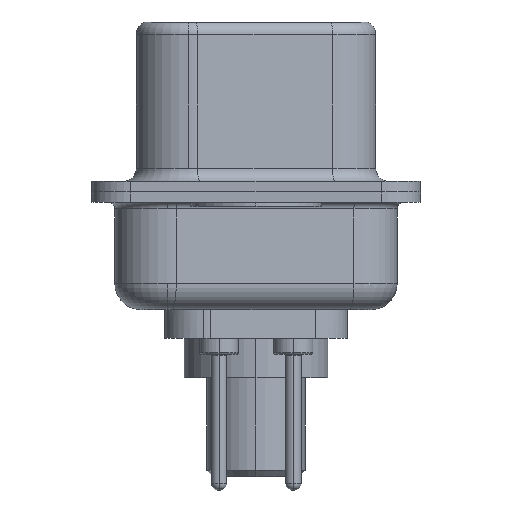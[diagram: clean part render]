
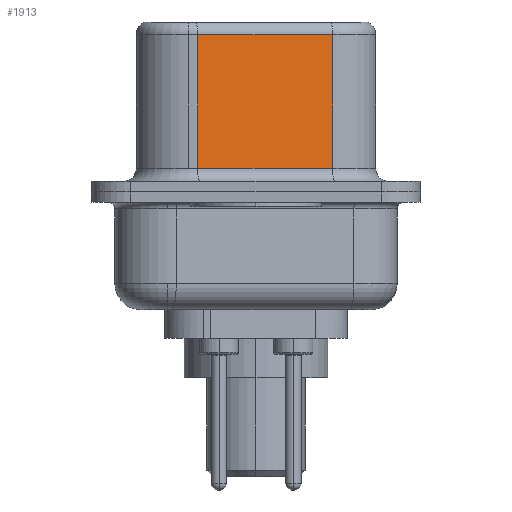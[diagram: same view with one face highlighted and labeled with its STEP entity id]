
A CAD part, left-side view. The second image highlights one B-rep face of the part: STEP entity #1913.
In plain terms, the highlighted planar face has unit normal (-0.985, -0.174, 0).
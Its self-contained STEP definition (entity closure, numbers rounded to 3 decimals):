
#334 = CARTESIAN_POINT ( 'NONE',  ( 3.67, 2.233, 6.02 ) ) ;
#497 = VECTOR ( 'NONE', #7940, 1000. ) ;
#1575 = AXIS2_PLACEMENT_3D ( 'NONE', #11495, #7559, #7485 ) ;
#1751 = VECTOR ( 'NONE', #2041, 1000. ) ;
#1789 = EDGE_CURVE ( 'NONE', #7858, #7710, #10670, .T. ) ;
#1827 = CARTESIAN_POINT ( 'NONE',  ( 4.58, -2.927, 0.9 ) ) ;
#1913 = ADVANCED_FACE ( 'NONE', ( #11664 ), #5556, .F. ) ;
#1963 = EDGE_CURVE ( 'NONE', #10136, #7858, #3935, .T. ) ;
#2041 = DIRECTION ( 'NONE',  ( 0., 0., -1. ) ) ;
#2373 = ORIENTED_EDGE ( 'NONE', *, *, #1963, .T. ) ;
#3032 = LINE ( 'NONE', #3913, #497 ) ;
#3173 = ORIENTED_EDGE ( 'NONE', *, *, #1789, .T. ) ;
#3664 = ORIENTED_EDGE ( 'NONE', *, *, #6048, .F. ) ;
#3708 = DIRECTION ( 'NONE',  ( -0.174, 0.985, 0. ) ) ;
#3713 = ORIENTED_EDGE ( 'NONE', *, *, #5382, .T. ) ;
#3913 = CARTESIAN_POINT ( 'NONE',  ( 4.58, -2.927, 6.52 ) ) ;
#3935 = LINE ( 'NONE', #6809, #1751 ) ;
#5369 = DIRECTION ( 'NONE',  ( 0.174, -0.985, 0. ) ) ;
#5382 = EDGE_CURVE ( 'NONE', #8556, #10136, #6538, .T. ) ;
#5556 = PLANE ( 'NONE',  #1575 ) ;
#6048 = EDGE_CURVE ( 'NONE', #8556, #7710, #3032, .T. ) ;
#6114 = CARTESIAN_POINT ( 'NONE',  ( 3.67, 2.233, 0.9 ) ) ;
#6538 = LINE ( 'NONE', #8829, #8767 ) ;
#6809 = CARTESIAN_POINT ( 'NONE',  ( 3.67, 2.233, 6.52 ) ) ;
#7485 = DIRECTION ( 'NONE',  ( -0.174, 0.985, 0. ) ) ;
#7559 = DIRECTION ( 'NONE',  ( 0.985, 0.174, 0. ) ) ;
#7710 = VERTEX_POINT ( 'NONE', #1827 ) ;
#7858 = VERTEX_POINT ( 'NONE', #6114 ) ;
#7940 = DIRECTION ( 'NONE',  ( 0., 0., -1. ) ) ;
#8373 = VECTOR ( 'NONE', #5369, 1000. ) ;
#8556 = VERTEX_POINT ( 'NONE', #9740 ) ;
#8767 = VECTOR ( 'NONE', #3708, 1000. ) ;
#8829 = CARTESIAN_POINT ( 'NONE',  ( 4.58, -2.927, 6.02 ) ) ;
#9374 = CARTESIAN_POINT ( 'NONE',  ( 4.58, -2.927, 0.9 ) ) ;
#9740 = CARTESIAN_POINT ( 'NONE',  ( 4.58, -2.927, 6.02 ) ) ;
#10136 = VERTEX_POINT ( 'NONE', #334 ) ;
#10670 = LINE ( 'NONE', #9374, #8373 ) ;
#11495 = CARTESIAN_POINT ( 'NONE',  ( 4.58, -2.927, 6.52 ) ) ;
#11664 = FACE_OUTER_BOUND ( 'NONE', #11992, .T. ) ;
#11992 = EDGE_LOOP ( 'NONE', ( #3664, #3713, #2373, #3173 ) ) ;
